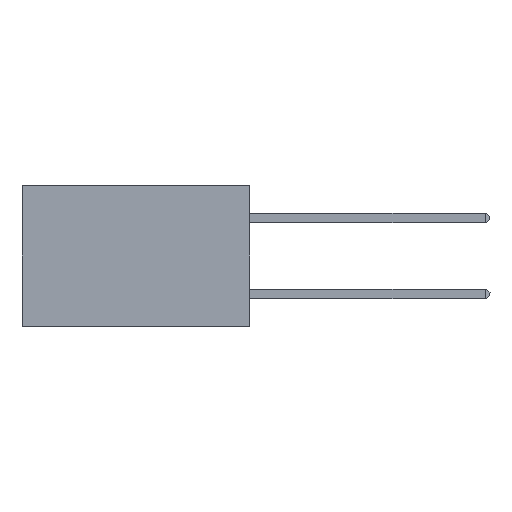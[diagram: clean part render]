
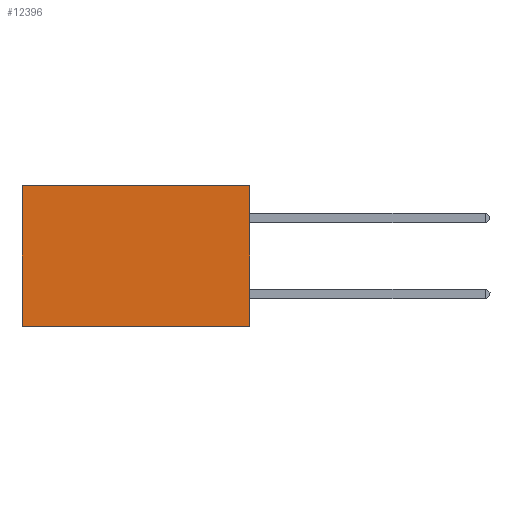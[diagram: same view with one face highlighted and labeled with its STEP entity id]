
A CAD part, left-side view. The second image highlights one B-rep face of the part: STEP entity #12396.
In plain terms, the highlighted planar face has unit normal (-1, 0, 0).
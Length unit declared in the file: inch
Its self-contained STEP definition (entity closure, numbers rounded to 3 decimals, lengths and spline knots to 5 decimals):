
#54 = DIRECTION ( 'NONE',  ( 1., 0., 0. ) ) ;
#318 = CARTESIAN_POINT ( 'NONE',  ( 0.2875, 0., -0.37 ) ) ;
#1004 = EDGE_CURVE ( 'NONE', #5427, #1231, #6107, .T. ) ;
#1231 = VERTEX_POINT ( 'NONE', #12590 ) ;
#2633 = CARTESIAN_POINT ( 'NONE',  ( 0.2875, 0., 0. ) ) ;
#3505 = LINE ( 'NONE', #5947, #12499 ) ;
#3526 = ORIENTED_EDGE ( 'NONE', *, *, #11047, .F. ) ;
#3958 = CARTESIAN_POINT ( 'NONE',  ( 0.2875, 0., 0. ) ) ;
#4470 = DIRECTION ( 'NONE',  ( 0., 0., -1. ) ) ;
#5069 = CARTESIAN_POINT ( 'NONE',  ( 0.2875, 0.6, 0. ) ) ;
#5393 = CARTESIAN_POINT ( 'NONE',  ( 0.2875, 0.6, 0. ) ) ;
#5427 = VERTEX_POINT ( 'NONE', #5069 ) ;
#5875 = LINE ( 'NONE', #7250, #11864 ) ;
#5947 = CARTESIAN_POINT ( 'NONE',  ( 0.2875, 0., -0.37 ) ) ;
#6107 = LINE ( 'NONE', #5393, #12949 ) ;
#6818 = DIRECTION ( 'NONE',  ( 0., 0., -1. ) ) ;
#7250 = CARTESIAN_POINT ( 'NONE',  ( 0.2875, 0., 0. ) ) ;
#7495 = VERTEX_POINT ( 'NONE', #318 ) ;
#7662 = ORIENTED_EDGE ( 'NONE', *, *, #15950, .T. ) ;
#7852 = ORIENTED_EDGE ( 'NONE', *, *, #1004, .T. ) ;
#8503 = LINE ( 'NONE', #13493, #8927 ) ;
#8927 = VECTOR ( 'NONE', #13550, 39.37008 ) ;
#10311 = AXIS2_PLACEMENT_3D ( 'NONE', #2633, #54, #6818 ) ;
#10544 = EDGE_CURVE ( 'NONE', #17311, #7495, #5875, .T. ) ;
#10572 = EDGE_LOOP ( 'NONE', ( #7852, #3526, #17056, #7662 ) ) ;
#11047 = EDGE_CURVE ( 'NONE', #7495, #1231, #3505, .T. ) ;
#11864 = VECTOR ( 'NONE', #4470, 39.37008 ) ;
#12396 = ADVANCED_FACE ( 'NONE', ( #16583 ), #16467, .F. ) ;
#12499 = VECTOR ( 'NONE', #15859, 39.37008 ) ;
#12590 = CARTESIAN_POINT ( 'NONE',  ( 0.2875, 0.6, -0.37 ) ) ;
#12949 = VECTOR ( 'NONE', #13466, 39.37008 ) ;
#13466 = DIRECTION ( 'NONE',  ( 0., 0., -1. ) ) ;
#13493 = CARTESIAN_POINT ( 'NONE',  ( 0.2875, 0., 0. ) ) ;
#13550 = DIRECTION ( 'NONE',  ( 0., 1., 0. ) ) ;
#15859 = DIRECTION ( 'NONE',  ( 0., 1., 0. ) ) ;
#15950 = EDGE_CURVE ( 'NONE', #17311, #5427, #8503, .T. ) ;
#16467 = PLANE ( 'NONE',  #10311 ) ;
#16583 = FACE_OUTER_BOUND ( 'NONE', #10572, .T. ) ;
#17056 = ORIENTED_EDGE ( 'NONE', *, *, #10544, .F. ) ;
#17311 = VERTEX_POINT ( 'NONE', #3958 ) ;
